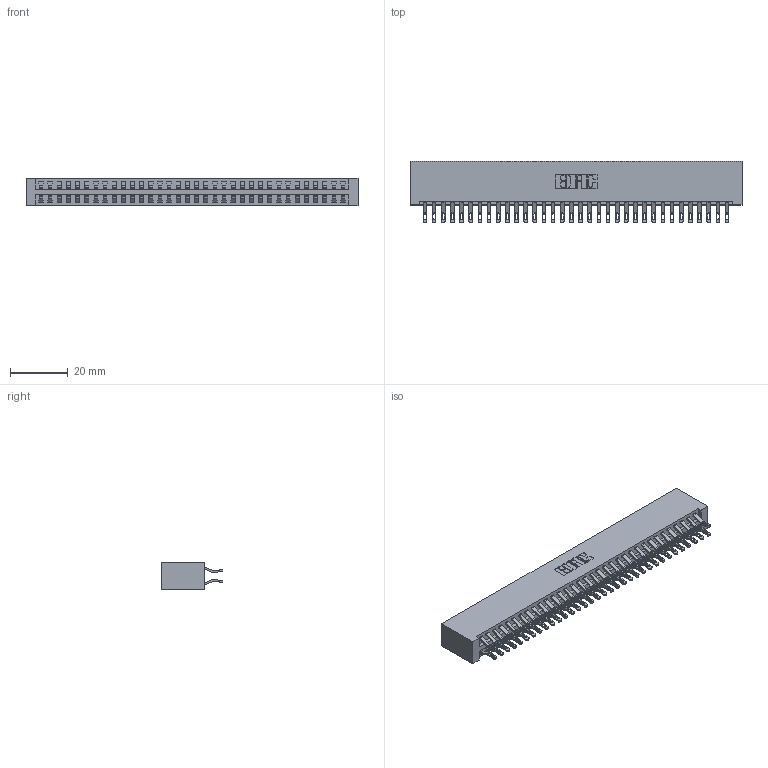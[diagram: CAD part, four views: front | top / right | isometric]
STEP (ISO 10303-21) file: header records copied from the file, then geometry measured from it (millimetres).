
FILE_DESCRIPTION (( 'STEP AP203' ), '1' );
FILE_NAME ('396-068-555-201.STEP', '2019-10-30T18:58:55', ( '' ), ( '' ), 'SwSTEP 2.0', 'SolidWorks 2016', '' );
FILE_SCHEMA (( 'CONFIG_CONTROL_DESIGN' ));
Length unit declared in the file: inch
Products named in the file (3): 396-068-555-201; 345-292-001_555 Tail; 346 Part_No Mounting Lugs
Assembly tree (69 placements, depth 2):
  396-068-555-201
    346 Part_No Mounting Lugs
    345-292-001_555 Tail  x68
Bounding box: 115.19 x 21.46 x 9.4 mm (x, y, z)
Volume: 11940.7 mm3; surface area: 17153.9 mm2
Topology: 69 solids, 69 shells, 4058 faces, 12749 edges, 8498 vertices
Faces by surface type: plane 2316, cylinder 1742
Entity records: 23315 total; most frequent: CARTESIAN_POINT 3886, ORIENTED_EDGE 3790, DIRECTION 3439, EDGE_CURVE 1895, VECTOR 1615, LINE 1615, VERTEX_POINT 1262, AXIS2_PLACEMENT_3D 912
